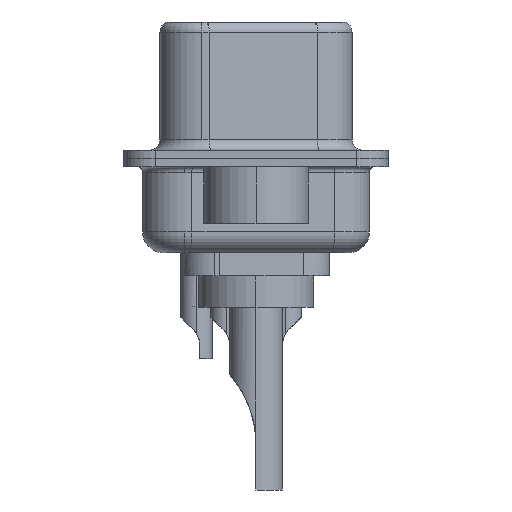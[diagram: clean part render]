
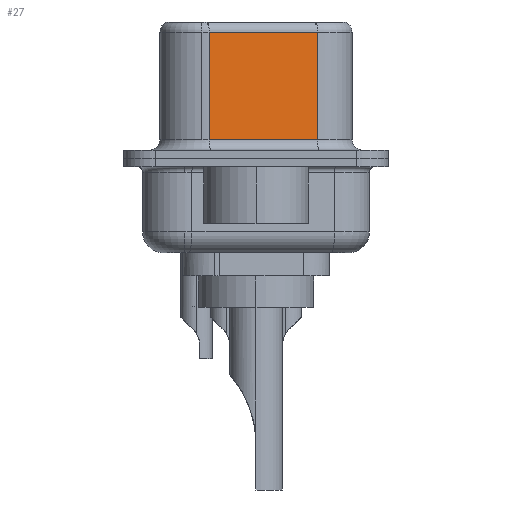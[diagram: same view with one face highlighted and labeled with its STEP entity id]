
A CAD part, left-side view. The second image highlights one B-rep face of the part: STEP entity #27.
In plain terms, the highlighted planar face has unit normal (-0.985, -0.174, 0).
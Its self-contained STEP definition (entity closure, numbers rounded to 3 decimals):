
#19 = ORIENTED_EDGE ( 'NONE', *, *, #14941, .T. ) ;
#27 = ADVANCED_FACE ( 'NONE', ( #11178 ), #7941, .F. ) ;
#199 = CARTESIAN_POINT ( 'NONE',  ( 3.67, 2.233, 6.02 ) ) ;
#238 = VERTEX_POINT ( 'NONE', #19473 ) ;
#3159 = VECTOR ( 'NONE', #9721, 1000. ) ;
#6359 = DIRECTION ( 'NONE',  ( 0., 0., -1. ) ) ;
#6773 = DIRECTION ( 'NONE',  ( 0.174, -0.985, 0. ) ) ;
#7204 = VECTOR ( 'NONE', #21368, 1000. ) ;
#7941 = PLANE ( 'NONE',  #8084 ) ;
#8084 = AXIS2_PLACEMENT_3D ( 'NONE', #21120, #11194, #9757 ) ;
#8956 = CARTESIAN_POINT ( 'NONE',  ( 3.67, 2.233, 0.9 ) ) ;
#9181 = CARTESIAN_POINT ( 'NONE',  ( 4.58, -2.927, 6.02 ) ) ;
#9721 = DIRECTION ( 'NONE',  ( 0., 0., -1. ) ) ;
#9741 = ORIENTED_EDGE ( 'NONE', *, *, #14446, .T. ) ;
#9757 = DIRECTION ( 'NONE',  ( -0.174, 0.985, 0. ) ) ;
#11178 = FACE_OUTER_BOUND ( 'NONE', #16666, .T. ) ;
#11194 = DIRECTION ( 'NONE',  ( 0.985, 0.174, 0. ) ) ;
#11833 = LINE ( 'NONE', #15114, #20821 ) ;
#12293 = EDGE_CURVE ( 'NONE', #12780, #238, #21414, .T. ) ;
#12423 = CARTESIAN_POINT ( 'NONE',  ( 4.58, -2.927, 6.02 ) ) ;
#12670 = VERTEX_POINT ( 'NONE', #8956 ) ;
#12749 = VERTEX_POINT ( 'NONE', #199 ) ;
#12780 = VERTEX_POINT ( 'NONE', #9181 ) ;
#13215 = CARTESIAN_POINT ( 'NONE',  ( 4.58, -2.927, 6.52 ) ) ;
#14446 = EDGE_CURVE ( 'NONE', #12780, #12749, #16580, .T. ) ;
#14941 = EDGE_CURVE ( 'NONE', #12670, #238, #21866, .T. ) ;
#15114 = CARTESIAN_POINT ( 'NONE',  ( 3.67, 2.233, 6.52 ) ) ;
#15407 = ORIENTED_EDGE ( 'NONE', *, *, #12293, .F. ) ;
#15525 = CARTESIAN_POINT ( 'NONE',  ( 4.58, -2.927, 0.9 ) ) ;
#16580 = LINE ( 'NONE', #12423, #7204 ) ;
#16666 = EDGE_LOOP ( 'NONE', ( #15407, #9741, #19148, #19 ) ) ;
#19148 = ORIENTED_EDGE ( 'NONE', *, *, #19454, .T. ) ;
#19454 = EDGE_CURVE ( 'NONE', #12749, #12670, #11833, .T. ) ;
#19473 = CARTESIAN_POINT ( 'NONE',  ( 4.58, -2.927, 0.9 ) ) ;
#20821 = VECTOR ( 'NONE', #6359, 1000. ) ;
#21120 = CARTESIAN_POINT ( 'NONE',  ( 4.58, -2.927, 6.52 ) ) ;
#21368 = DIRECTION ( 'NONE',  ( -0.174, 0.985, 0. ) ) ;
#21414 = LINE ( 'NONE', #13215, #3159 ) ;
#21866 = LINE ( 'NONE', #15525, #22419 ) ;
#22419 = VECTOR ( 'NONE', #6773, 1000. ) ;
